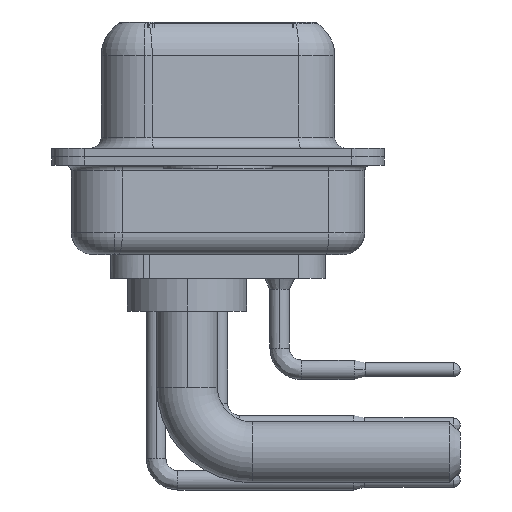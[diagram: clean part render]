
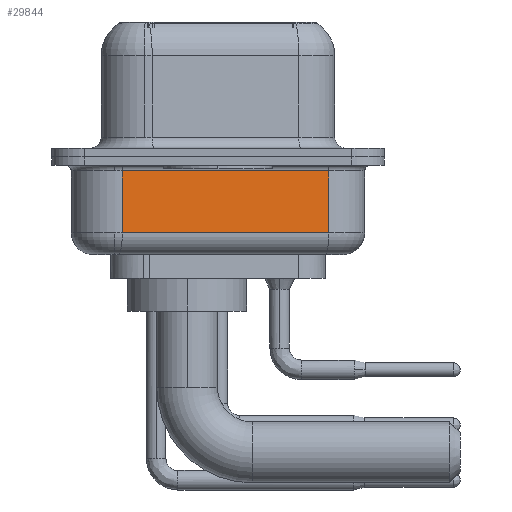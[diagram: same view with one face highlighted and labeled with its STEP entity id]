
A CAD part, left-side view. The second image highlights one B-rep face of the part: STEP entity #29844.
In plain terms, the highlighted planar face has unit normal (-0.985, -0.174, 0).
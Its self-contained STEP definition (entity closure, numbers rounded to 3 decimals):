
#108 = ORIENTED_EDGE ( 'NONE', *, *, #28017, .T. ) ;
#1960 = EDGE_CURVE ( 'NONE', #28545, #12461, #15633, .T. ) ;
#2709 = CARTESIAN_POINT ( 'NONE',  ( 2.93, 4.403, -3.5 ) ) ;
#3462 = CARTESIAN_POINT ( 'NONE',  ( 2.93, 4.403, -4.5 ) ) ;
#3622 = DIRECTION ( 'NONE',  ( -0.174, 0.985, 0. ) ) ;
#4111 = CARTESIAN_POINT ( 'NONE',  ( 2.93, 4.403, -0.65 ) ) ;
#6121 = LINE ( 'NONE', #19998, #18258 ) ;
#6411 = DIRECTION ( 'NONE',  ( 0.985, 0.174, 0. ) ) ;
#8268 = CARTESIAN_POINT ( 'NONE',  ( 4.605, -5.097, -3.5 ) ) ;
#8731 = FACE_OUTER_BOUND ( 'NONE', #17974, .T. ) ;
#9201 = VECTOR ( 'NONE', #15937, 1000. ) ;
#9565 = VECTOR ( 'NONE', #23090, 1000. ) ;
#9996 = CARTESIAN_POINT ( 'NONE',  ( 4.605, -5.097, -0.65 ) ) ;
#10616 = PLANE ( 'NONE',  #14628 ) ;
#11701 = CARTESIAN_POINT ( 'NONE',  ( 2.93, 4.403, -4.5 ) ) ;
#12461 = VERTEX_POINT ( 'NONE', #9996 ) ;
#12942 = VERTEX_POINT ( 'NONE', #18195 ) ;
#13283 = LINE ( 'NONE', #4111, #9565 ) ;
#13518 = VERTEX_POINT ( 'NONE', #2709 ) ;
#13805 = EDGE_CURVE ( 'NONE', #13518, #28545, #6121, .T. ) ;
#13953 = VECTOR ( 'NONE', #23688, 1000. ) ;
#14188 = LINE ( 'NONE', #11701, #13953 ) ;
#14628 = AXIS2_PLACEMENT_3D ( 'NONE', #3462, #6411, #3622 ) ;
#15218 = ORIENTED_EDGE ( 'NONE', *, *, #26275, .F. ) ;
#15633 = LINE ( 'NONE', #17828, #9201 ) ;
#15937 = DIRECTION ( 'NONE',  ( 0., 0., 1. ) ) ;
#17828 = CARTESIAN_POINT ( 'NONE',  ( 4.605, -5.097, -4.5 ) ) ;
#17974 = EDGE_LOOP ( 'NONE', ( #15218, #27459, #20235, #108 ) ) ;
#18195 = CARTESIAN_POINT ( 'NONE',  ( 2.93, 4.403, -0.65 ) ) ;
#18258 = VECTOR ( 'NONE', #29457, 1000. ) ;
#19998 = CARTESIAN_POINT ( 'NONE',  ( 2.93, 4.403, -3.5 ) ) ;
#20235 = ORIENTED_EDGE ( 'NONE', *, *, #1960, .T. ) ;
#23090 = DIRECTION ( 'NONE',  ( -0.174, 0.985, 0. ) ) ;
#23688 = DIRECTION ( 'NONE',  ( 0., 0., 1. ) ) ;
#26275 = EDGE_CURVE ( 'NONE', #13518, #12942, #14188, .T. ) ;
#27459 = ORIENTED_EDGE ( 'NONE', *, *, #13805, .T. ) ;
#28017 = EDGE_CURVE ( 'NONE', #12461, #12942, #13283, .T. ) ;
#28545 = VERTEX_POINT ( 'NONE', #8268 ) ;
#29457 = DIRECTION ( 'NONE',  ( 0.174, -0.985, 0. ) ) ;
#29844 = ADVANCED_FACE ( 'NONE', ( #8731 ), #10616, .F. ) ;
